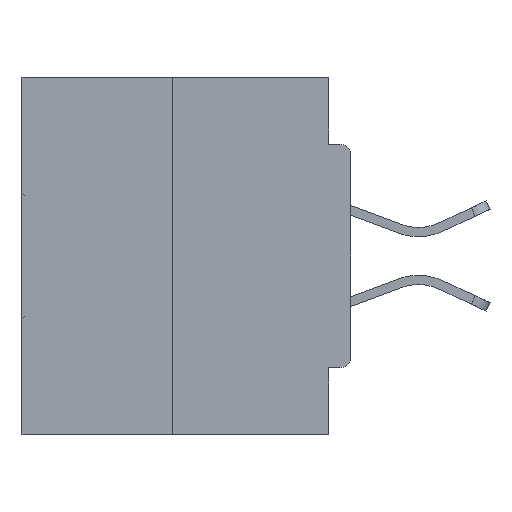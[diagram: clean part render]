
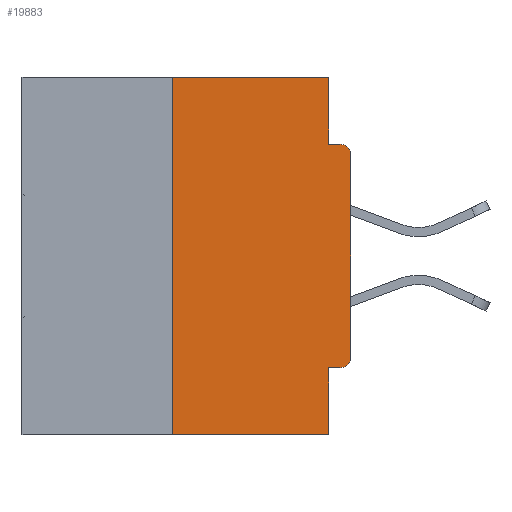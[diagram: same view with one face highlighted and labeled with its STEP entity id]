
A CAD part, left-side view. The second image highlights one B-rep face of the part: STEP entity #19883.
In plain terms, the highlighted planar face has unit normal (-1, 0, 0).
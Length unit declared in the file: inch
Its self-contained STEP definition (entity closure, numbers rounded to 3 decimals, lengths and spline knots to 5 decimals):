
#199 = DIRECTION ( 'NONE',  ( 0., 0., 1. ) ) ;
#440 = CARTESIAN_POINT ( 'NONE',  ( 0., 0.015, -0.1085 ) ) ;
#1092 = VERTEX_POINT ( 'NONE', #14702 ) ;
#1395 = VECTOR ( 'NONE', #21529, 39.37008 ) ;
#2498 = CIRCLE ( 'NONE', #19230, 0.015 ) ;
#2524 = CIRCLE ( 'NONE', #19981, 0.015 ) ;
#3133 = VERTEX_POINT ( 'NONE', #15847 ) ;
#3506 = VECTOR ( 'NONE', #12872, 39.37008 ) ;
#3890 = VERTEX_POINT ( 'NONE', #11077 ) ;
#4414 = EDGE_CURVE ( 'NONE', #18372, #5388, #11790, .T. ) ;
#4716 = VECTOR ( 'NONE', #14558, 39.37008 ) ;
#5166 = EDGE_CURVE ( 'NONE', #39916, #6890, #38026, .T. ) ;
#5388 = VERTEX_POINT ( 'NONE', #6269 ) ;
#6269 = CARTESIAN_POINT ( 'NONE',  ( 0., 0.031, -0.5 ) ) ;
#6700 = CARTESIAN_POINT ( 'NONE',  ( 0., 0.031, 0. ) ) ;
#6890 = VERTEX_POINT ( 'NONE', #38904 ) ;
#7649 = DIRECTION ( 'NONE',  ( 0., 0., -1. ) ) ;
#8326 = DIRECTION ( 'NONE',  ( 0., 0., -1. ) ) ;
#8429 = ORIENTED_EDGE ( 'NONE', *, *, #18248, .T. ) ;
#9289 = VECTOR ( 'NONE', #33737, 39.37008 ) ;
#9807 = CARTESIAN_POINT ( 'NONE',  ( 0., 0.25, 0. ) ) ;
#9855 = CARTESIAN_POINT ( 'NONE',  ( 0., 0.031, -0.0935 ) ) ;
#9987 = VECTOR ( 'NONE', #29232, 39.37008 ) ;
#10663 = EDGE_CURVE ( 'NONE', #3133, #14206, #2498, .T. ) ;
#11077 = CARTESIAN_POINT ( 'NONE',  ( 0., 0., -0.1085 ) ) ;
#11154 = ORIENTED_EDGE ( 'NONE', *, *, #14360, .F. ) ;
#11790 = LINE ( 'NONE', #30285, #9289 ) ;
#12802 = EDGE_CURVE ( 'NONE', #1092, #5388, #23695, .T. ) ;
#12872 = DIRECTION ( 'NONE',  ( 0., 0., -1. ) ) ;
#12883 = AXIS2_PLACEMENT_3D ( 'NONE', #27794, #30990, #8326 ) ;
#14205 = ORIENTED_EDGE ( 'NONE', *, *, #31601, .F. ) ;
#14206 = VERTEX_POINT ( 'NONE', #37738 ) ;
#14360 = EDGE_CURVE ( 'NONE', #14492, #30117, #19388, .T. ) ;
#14492 = VERTEX_POINT ( 'NONE', #9807 ) ;
#14558 = DIRECTION ( 'NONE',  ( 0., 0., -1. ) ) ;
#14594 = EDGE_CURVE ( 'NONE', #18372, #14492, #14906, .T. ) ;
#14702 = CARTESIAN_POINT ( 'NONE',  ( 0., 0.031, -0.4065 ) ) ;
#14901 = EDGE_CURVE ( 'NONE', #3133, #1092, #31335, .T. ) ;
#14906 = LINE ( 'NONE', #20324, #9987 ) ;
#15139 = CARTESIAN_POINT ( 'NONE',  ( 0., 0.46, 0. ) ) ;
#15847 = CARTESIAN_POINT ( 'NONE',  ( 0., 0.015, -0.4065 ) ) ;
#18170 = PLANE ( 'NONE',  #12883 ) ;
#18248 = EDGE_CURVE ( 'NONE', #3890, #6890, #2524, .T. ) ;
#18372 = VERTEX_POINT ( 'NONE', #30937 ) ;
#19230 = AXIS2_PLACEMENT_3D ( 'NONE', #39605, #36577, #7649 ) ;
#19388 = LINE ( 'NONE', #15139, #1395 ) ;
#19883 = ADVANCED_FACE ( 'NONE', ( #36826 ), #18170, .F. ) ;
#19981 = AXIS2_PLACEMENT_3D ( 'NONE', #440, #22620, #25809 ) ;
#19990 = ORIENTED_EDGE ( 'NONE', *, *, #39567, .T. ) ;
#20324 = CARTESIAN_POINT ( 'NONE',  ( 0., 0.25, 0. ) ) ;
#21227 = CARTESIAN_POINT ( 'NONE',  ( 0., 0.031, -0.5 ) ) ;
#21529 = DIRECTION ( 'NONE',  ( 0., -1., 0. ) ) ;
#22620 = DIRECTION ( 'NONE',  ( -1., 0., 0. ) ) ;
#23695 = LINE ( 'NONE', #21227, #4716 ) ;
#24062 = ORIENTED_EDGE ( 'NONE', *, *, #10663, .T. ) ;
#24186 = DIRECTION ( 'NONE',  ( 0., -1., 0. ) ) ;
#25809 = DIRECTION ( 'NONE',  ( 0., 0., -1. ) ) ;
#26268 = ORIENTED_EDGE ( 'NONE', *, *, #4414, .T. ) ;
#27249 = DIRECTION ( 'NONE',  ( 0., 1., 0. ) ) ;
#27502 = CARTESIAN_POINT ( 'NONE',  ( 0., 0., -0.4065 ) ) ;
#27794 = CARTESIAN_POINT ( 'NONE',  ( 0., 0.46, 0. ) ) ;
#28929 = LINE ( 'NONE', #32479, #3506 ) ;
#29232 = DIRECTION ( 'NONE',  ( 0., 0., 1. ) ) ;
#30012 = VECTOR ( 'NONE', #199, 39.37008 ) ;
#30117 = VERTEX_POINT ( 'NONE', #6700 ) ;
#30285 = CARTESIAN_POINT ( 'NONE',  ( 0., 0.46, -0.5 ) ) ;
#30574 = ORIENTED_EDGE ( 'NONE', *, *, #5166, .F. ) ;
#30937 = CARTESIAN_POINT ( 'NONE',  ( 0., 0.25, -0.5 ) ) ;
#30990 = DIRECTION ( 'NONE',  ( 1., 0., 0. ) ) ;
#31028 = ORIENTED_EDGE ( 'NONE', *, *, #14594, .F. ) ;
#31335 = LINE ( 'NONE', #27502, #38801 ) ;
#31601 = EDGE_CURVE ( 'NONE', #30117, #39916, #28929, .T. ) ;
#32479 = CARTESIAN_POINT ( 'NONE',  ( 0., 0.031, 0. ) ) ;
#33737 = DIRECTION ( 'NONE',  ( 0., -1., 0. ) ) ;
#35306 = EDGE_LOOP ( 'NONE', ( #11154, #31028, #26268, #39038, #40430, #24062, #19990, #8429, #30574, #14205 ) ) ;
#36518 = LINE ( 'NONE', #38243, #30012 ) ;
#36576 = VECTOR ( 'NONE', #24186, 39.37008 ) ;
#36577 = DIRECTION ( 'NONE',  ( -1., 0., 0. ) ) ;
#36826 = FACE_OUTER_BOUND ( 'NONE', #35306, .T. ) ;
#36968 = CARTESIAN_POINT ( 'NONE',  ( 0., 0., -0.0935 ) ) ;
#37738 = CARTESIAN_POINT ( 'NONE',  ( 0., 0., -0.3915 ) ) ;
#38026 = LINE ( 'NONE', #36968, #36576 ) ;
#38243 = CARTESIAN_POINT ( 'NONE',  ( 0., 0., 0. ) ) ;
#38801 = VECTOR ( 'NONE', #27249, 39.37008 ) ;
#38904 = CARTESIAN_POINT ( 'NONE',  ( 0., 0.015, -0.0935 ) ) ;
#39038 = ORIENTED_EDGE ( 'NONE', *, *, #12802, .F. ) ;
#39567 = EDGE_CURVE ( 'NONE', #14206, #3890, #36518, .T. ) ;
#39605 = CARTESIAN_POINT ( 'NONE',  ( 0., 0.015, -0.3915 ) ) ;
#39916 = VERTEX_POINT ( 'NONE', #9855 ) ;
#40430 = ORIENTED_EDGE ( 'NONE', *, *, #14901, .F. ) ;
